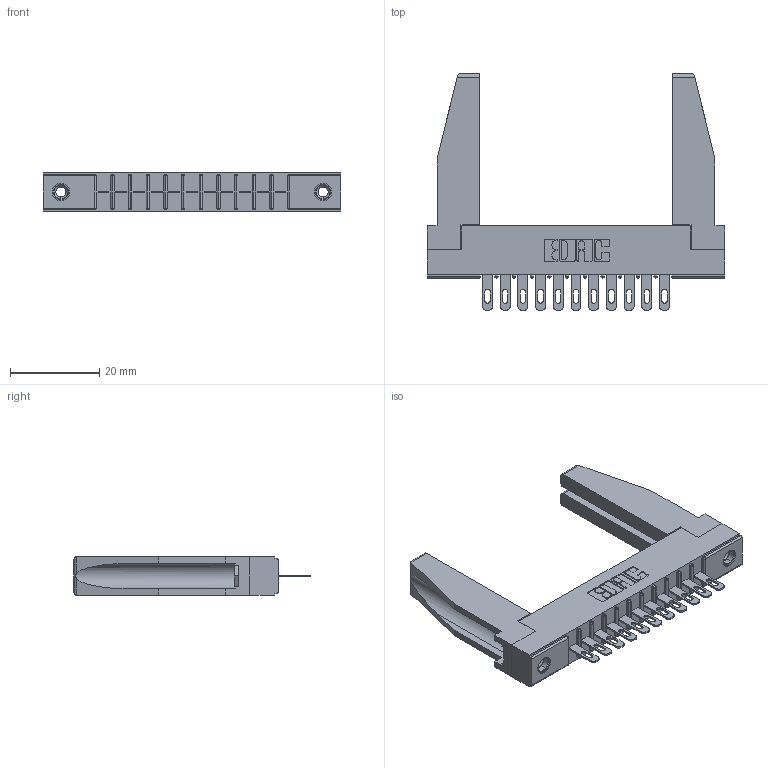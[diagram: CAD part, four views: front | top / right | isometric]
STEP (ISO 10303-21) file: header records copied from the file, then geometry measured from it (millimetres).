
FILE_DESCRIPTION (( 'STEP AP203' ), '1' );
FILE_NAME ('316-011-500-178.STEP', '2018-07-31T00:15:11', ( '' ), ( '' ), 'SwSTEP 2.0', 'SolidWorks 2016', '' );
FILE_SCHEMA (( 'CONFIG_CONTROL_DESIGN' ));
Length unit declared in the file: inch
Products named in the file (5): 345-250-001_345-250-001-102; 307-220-078; 316-011-500-178; 306 Part_.156 Dia; 306-290-001_100
Assembly tree (16 placements, depth 2):
  316-011-500-178
    306 Part_.156 Dia
    306-290-001_100  x11
    345-250-001_345-250-001-102  x2
    307-220-078  x2
Bounding box: 66.6 x 52.91 x 8.71 mm (x, y, z)
Volume: 8539 mm3; surface area: 10369 mm2
Topology: 16 solids, 16 shells, 1082 faces, 3011 edges, 1938 vertices
Faces by surface type: plane 702, cylinder 320, sphere 44, cone 12, torus 4
Entity records: 16877 total; most frequent: CARTESIAN_POINT 2830, ORIENTED_EDGE 2760, DIRECTION 2746, EDGE_CURVE 1380, VECTOR 1062, LINE 1062, VERTEX_POINT 884, AXIS2_PLACEMENT_3D 842
